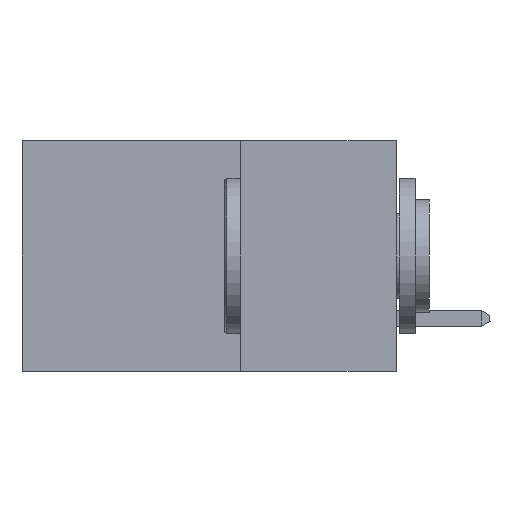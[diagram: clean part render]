
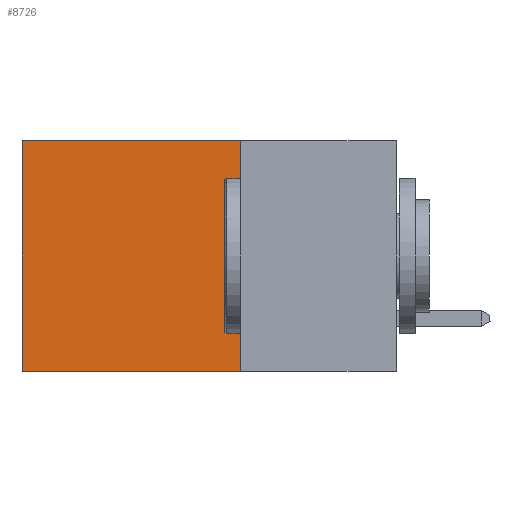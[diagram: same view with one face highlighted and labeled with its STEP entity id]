
A CAD part, left-side view. The second image highlights one B-rep face of the part: STEP entity #8726.
In plain terms, the highlighted planar face has unit normal (-1, 0, 0).
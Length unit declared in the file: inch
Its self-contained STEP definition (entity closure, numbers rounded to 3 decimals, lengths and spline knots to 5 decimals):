
#629 = DIRECTION ( 'NONE',  ( 0., 0., -1. ) ) ;
#727 = PLANE ( 'NONE',  #6385 ) ;
#902 = CARTESIAN_POINT ( 'NONE',  ( 0.298, 0.6, 0. ) ) ;
#1297 = ORIENTED_EDGE ( 'NONE', *, *, #8040, .T. ) ;
#1325 = CARTESIAN_POINT ( 'NONE',  ( 0.298, 0.25, 0. ) ) ;
#1954 = ORIENTED_EDGE ( 'NONE', *, *, #6157, .F. ) ;
#2188 = DIRECTION ( 'NONE',  ( 0., 1., 0. ) ) ;
#2500 = VERTEX_POINT ( 'NONE', #7956 ) ;
#2529 = EDGE_CURVE ( 'NONE', #3577, #2500, #6677, .T. ) ;
#2647 = VECTOR ( 'NONE', #2188, 39.37008 ) ;
#2724 = DIRECTION ( 'NONE',  ( 0., 0., -1. ) ) ;
#3577 = VERTEX_POINT ( 'NONE', #9518 ) ;
#4201 = DIRECTION ( 'NONE',  ( 0., 1., 0. ) ) ;
#5259 = CARTESIAN_POINT ( 'NONE',  ( 0.298, 0.25, -0.37 ) ) ;
#5651 = LINE ( 'NONE', #5259, #9382 ) ;
#5834 = ORIENTED_EDGE ( 'NONE', *, *, #2529, .T. ) ;
#6004 = FACE_OUTER_BOUND ( 'NONE', #6923, .T. ) ;
#6157 = EDGE_CURVE ( 'NONE', #7073, #11659, #6867, .T. ) ;
#6366 = CARTESIAN_POINT ( 'NONE',  ( 0.298, 0.25, 0. ) ) ;
#6385 = AXIS2_PLACEMENT_3D ( 'NONE', #9750, #6610, #2724 ) ;
#6496 = LINE ( 'NONE', #1325, #2647 ) ;
#6552 = CARTESIAN_POINT ( 'NONE',  ( 0.298, 0.25, 0. ) ) ;
#6581 = ORIENTED_EDGE ( 'NONE', *, *, #12251, .F. ) ;
#6610 = DIRECTION ( 'NONE',  ( 1., 0., 0. ) ) ;
#6677 = LINE ( 'NONE', #902, #11828 ) ;
#6867 = LINE ( 'NONE', #6552, #11862 ) ;
#6923 = EDGE_LOOP ( 'NONE', ( #5834, #6581, #1954, #1297 ) ) ;
#7073 = VERTEX_POINT ( 'NONE', #6366 ) ;
#7956 = CARTESIAN_POINT ( 'NONE',  ( 0.298, 0.6, -0.37 ) ) ;
#8040 = EDGE_CURVE ( 'NONE', #7073, #3577, #6496, .T. ) ;
#8726 = ADVANCED_FACE ( 'NONE', ( #6004 ), #727, .F. ) ;
#9382 = VECTOR ( 'NONE', #4201, 39.37008 ) ;
#9518 = CARTESIAN_POINT ( 'NONE',  ( 0.298, 0.6, 0. ) ) ;
#9750 = CARTESIAN_POINT ( 'NONE',  ( 0.298, 0.25, 0. ) ) ;
#11659 = VERTEX_POINT ( 'NONE', #12740 ) ;
#11828 = VECTOR ( 'NONE', #12806, 39.37008 ) ;
#11862 = VECTOR ( 'NONE', #629, 39.37008 ) ;
#12251 = EDGE_CURVE ( 'NONE', #11659, #2500, #5651, .T. ) ;
#12740 = CARTESIAN_POINT ( 'NONE',  ( 0.298, 0.25, -0.37 ) ) ;
#12806 = DIRECTION ( 'NONE',  ( 0., 0., -1. ) ) ;
